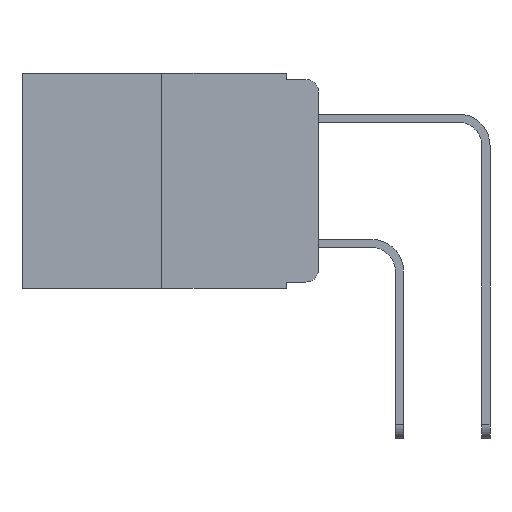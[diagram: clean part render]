
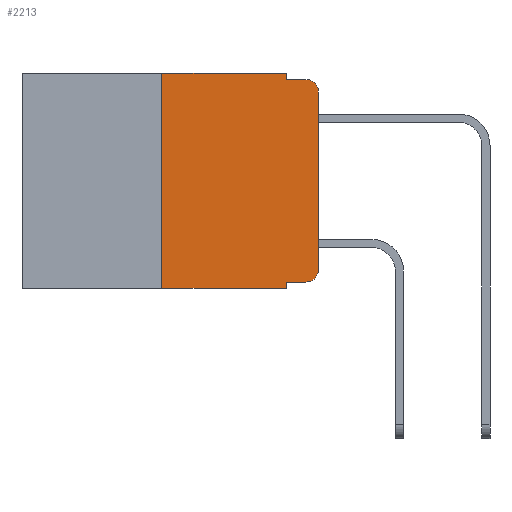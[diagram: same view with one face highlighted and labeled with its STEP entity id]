
A CAD part, left-side view. The second image highlights one B-rep face of the part: STEP entity #2213.
In plain terms, the highlighted planar face has unit normal (-1, 0, 0).
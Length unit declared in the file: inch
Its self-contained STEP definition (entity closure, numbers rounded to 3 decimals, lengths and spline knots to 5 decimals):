
#132 = VERTEX_POINT ( 'NONE', #9311 ) ;
#483 = VERTEX_POINT ( 'NONE', #10046 ) ;
#647 = EDGE_CURVE ( 'NONE', #483, #8102, #6504, .T. ) ;
#684 = ORIENTED_EDGE ( 'NONE', *, *, #10761, .T. ) ;
#936 = VECTOR ( 'NONE', #9787, 39.37008 ) ;
#1152 = DIRECTION ( 'NONE',  ( 0., 0., -1. ) ) ;
#1165 = VECTOR ( 'NONE', #1152, 39.37008 ) ;
#1173 = LINE ( 'NONE', #6482, #3256 ) ;
#1275 = CARTESIAN_POINT ( 'NONE',  ( 0., 0.051, 0. ) ) ;
#1308 = CARTESIAN_POINT ( 'NONE',  ( 0., 0., -0.03 ) ) ;
#1324 = CARTESIAN_POINT ( 'NONE',  ( 0., 0.051, -0.01 ) ) ;
#1508 = DIRECTION ( 'NONE',  ( 0., 0., -1. ) ) ;
#1589 = VECTOR ( 'NONE', #4736, 39.37008 ) ;
#1678 = CARTESIAN_POINT ( 'NONE',  ( 0., 0.473, 0. ) ) ;
#1722 = ORIENTED_EDGE ( 'NONE', *, *, #10919, .F. ) ;
#2069 = FACE_OUTER_BOUND ( 'NONE', #4175, .T. ) ;
#2120 = ORIENTED_EDGE ( 'NONE', *, *, #3169, .T. ) ;
#2158 = ORIENTED_EDGE ( 'NONE', *, *, #5526, .F. ) ;
#2213 = ADVANCED_FACE ( 'NONE', ( #2069 ), #5535, .F. ) ;
#2345 = CARTESIAN_POINT ( 'NONE',  ( 0., 0.25, 0. ) ) ;
#2511 = CARTESIAN_POINT ( 'NONE',  ( 0., 0.02, -0.313 ) ) ;
#2526 = DIRECTION ( 'NONE',  ( -1., 0., 0. ) ) ;
#2540 = DIRECTION ( 'NONE',  ( 0., 0., -1. ) ) ;
#2808 = LINE ( 'NONE', #9451, #9242 ) ;
#2884 = CIRCLE ( 'NONE', #4809, 0.02 ) ;
#2954 = VERTEX_POINT ( 'NONE', #3447 ) ;
#3000 = EDGE_CURVE ( 'NONE', #3574, #483, #2884, .T. ) ;
#3169 = EDGE_CURVE ( 'NONE', #2954, #3574, #7814, .T. ) ;
#3242 = LINE ( 'NONE', #1275, #1165 ) ;
#3256 = VECTOR ( 'NONE', #4945, 39.37008 ) ;
#3279 = VERTEX_POINT ( 'NONE', #5699 ) ;
#3447 = CARTESIAN_POINT ( 'NONE',  ( 0., 0.051, -0.333 ) ) ;
#3574 = VERTEX_POINT ( 'NONE', #8814 ) ;
#3667 = DIRECTION ( 'NONE',  ( 0., 0., 1. ) ) ;
#3907 = LINE ( 'NONE', #9285, #7333 ) ;
#3955 = LINE ( 'NONE', #8909, #1589 ) ;
#4104 = CARTESIAN_POINT ( 'NONE',  ( 0., 0.051, 0. ) ) ;
#4175 = EDGE_LOOP ( 'NONE', ( #7098, #8261, #6352, #1722, #5049, #6008, #684, #2158, #2120, #6719 ) ) ;
#4209 = VERTEX_POINT ( 'NONE', #4104 ) ;
#4253 = VECTOR ( 'NONE', #6104, 39.37008 ) ;
#4281 = AXIS2_PLACEMENT_3D ( 'NONE', #1678, #5314, #1508 ) ;
#4445 = CARTESIAN_POINT ( 'NONE',  ( 0., 0.02, -0.03 ) ) ;
#4736 = DIRECTION ( 'NONE',  ( 0., 0., -1. ) ) ;
#4809 = AXIS2_PLACEMENT_3D ( 'NONE', #2511, #2526, #2540 ) ;
#4945 = DIRECTION ( 'NONE',  ( 0., -1., 0. ) ) ;
#5049 = ORIENTED_EDGE ( 'NONE', *, *, #6208, .F. ) ;
#5314 = DIRECTION ( 'NONE',  ( 1., 0., 0. ) ) ;
#5526 = EDGE_CURVE ( 'NONE', #2954, #3279, #3242, .T. ) ;
#5535 = PLANE ( 'NONE',  #4281 ) ;
#5699 = CARTESIAN_POINT ( 'NONE',  ( 0., 0.051, -0.343 ) ) ;
#5775 = DIRECTION ( 'NONE',  ( -1., 0., 0. ) ) ;
#5889 = EDGE_CURVE ( 'NONE', #8102, #132, #10363, .T. ) ;
#5960 = VECTOR ( 'NONE', #3667, 39.37008 ) ;
#6008 = ORIENTED_EDGE ( 'NONE', *, *, #7182, .F. ) ;
#6104 = DIRECTION ( 'NONE',  ( 0., 0., 1. ) ) ;
#6193 = DIRECTION ( 'NONE',  ( 0., -1., 0. ) ) ;
#6208 = EDGE_CURVE ( 'NONE', #8476, #4209, #2808, .T. ) ;
#6211 = LINE ( 'NONE', #2345, #5960 ) ;
#6352 = ORIENTED_EDGE ( 'NONE', *, *, #7528, .F. ) ;
#6482 = CARTESIAN_POINT ( 'NONE',  ( 0., 0.473, -0.343 ) ) ;
#6504 = LINE ( 'NONE', #10891, #4253 ) ;
#6719 = ORIENTED_EDGE ( 'NONE', *, *, #3000, .T. ) ;
#7098 = ORIENTED_EDGE ( 'NONE', *, *, #647, .T. ) ;
#7182 = EDGE_CURVE ( 'NONE', #7682, #8476, #6211, .T. ) ;
#7333 = VECTOR ( 'NONE', #6193, 39.37008 ) ;
#7431 = DIRECTION ( 'NONE',  ( 0., -1., 0. ) ) ;
#7528 = EDGE_CURVE ( 'NONE', #7572, #132, #3907, .T. ) ;
#7572 = VERTEX_POINT ( 'NONE', #1324 ) ;
#7682 = VERTEX_POINT ( 'NONE', #9682 ) ;
#7814 = LINE ( 'NONE', #9784, #936 ) ;
#7816 = CARTESIAN_POINT ( 'NONE',  ( 0., 0.25, 0. ) ) ;
#8102 = VERTEX_POINT ( 'NONE', #1308 ) ;
#8261 = ORIENTED_EDGE ( 'NONE', *, *, #5889, .T. ) ;
#8476 = VERTEX_POINT ( 'NONE', #7816 ) ;
#8814 = CARTESIAN_POINT ( 'NONE',  ( 0., 0.02, -0.333 ) ) ;
#8909 = CARTESIAN_POINT ( 'NONE',  ( 0., 0.051, 0. ) ) ;
#9128 = DIRECTION ( 'NONE',  ( 0., 0., -1. ) ) ;
#9242 = VECTOR ( 'NONE', #7431, 39.37008 ) ;
#9285 = CARTESIAN_POINT ( 'NONE',  ( 0., 0.051, -0.01 ) ) ;
#9311 = CARTESIAN_POINT ( 'NONE',  ( 0., 0.02, -0.01 ) ) ;
#9451 = CARTESIAN_POINT ( 'NONE',  ( 0., 0.473, 0. ) ) ;
#9682 = CARTESIAN_POINT ( 'NONE',  ( 0., 0.25, -0.343 ) ) ;
#9784 = CARTESIAN_POINT ( 'NONE',  ( 0., 0.051, -0.333 ) ) ;
#9787 = DIRECTION ( 'NONE',  ( 0., -1., 0. ) ) ;
#10046 = CARTESIAN_POINT ( 'NONE',  ( 0., 0., -0.313 ) ) ;
#10363 = CIRCLE ( 'NONE', #10407, 0.02 ) ;
#10407 = AXIS2_PLACEMENT_3D ( 'NONE', #4445, #5775, #9128 ) ;
#10761 = EDGE_CURVE ( 'NONE', #7682, #3279, #1173, .T. ) ;
#10891 = CARTESIAN_POINT ( 'NONE',  ( 0., 0., 0. ) ) ;
#10919 = EDGE_CURVE ( 'NONE', #4209, #7572, #3955, .T. ) ;
